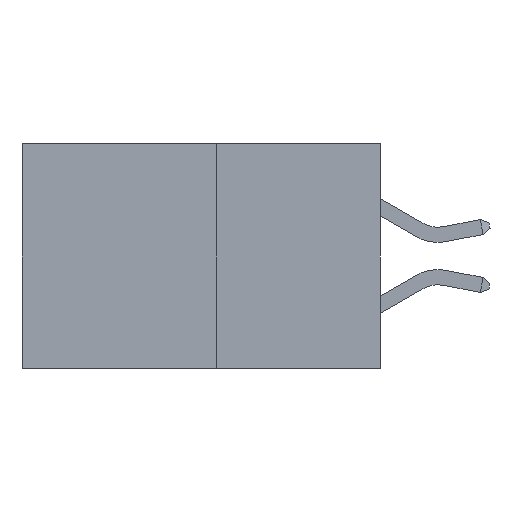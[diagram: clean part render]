
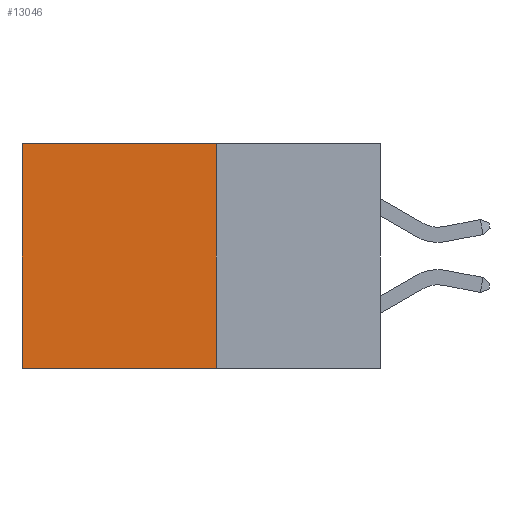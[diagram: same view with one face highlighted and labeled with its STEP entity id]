
A CAD part, left-side view. The second image highlights one B-rep face of the part: STEP entity #13046.
In plain terms, the highlighted planar face has unit normal (-1, 0, 0).
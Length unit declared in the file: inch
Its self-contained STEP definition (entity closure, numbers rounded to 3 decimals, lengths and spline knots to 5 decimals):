
#622 = LINE ( 'NONE', #9996, #13146 ) ;
#1147 = DIRECTION ( 'NONE',  ( 0., 0., -1. ) ) ;
#2276 = AXIS2_PLACEMENT_3D ( 'NONE', #18477, #28345, #23490 ) ;
#3434 = CARTESIAN_POINT ( 'NONE',  ( 0.277, 0.59, -0.37 ) ) ;
#4734 = VECTOR ( 'NONE', #1147, 39.37008 ) ;
#7025 = VERTEX_POINT ( 'NONE', #16132 ) ;
#7640 = ORIENTED_EDGE ( 'NONE', *, *, #30612, .F. ) ;
#9273 = CARTESIAN_POINT ( 'NONE',  ( 0.277, 0.27, 0. ) ) ;
#9689 = VERTEX_POINT ( 'NONE', #9793 ) ;
#9793 = CARTESIAN_POINT ( 'NONE',  ( 0.277, 0.59, 0. ) ) ;
#9996 = CARTESIAN_POINT ( 'NONE',  ( 0.277, 0.27, -0.37 ) ) ;
#10485 = CARTESIAN_POINT ( 'NONE',  ( 0.277, 0.27, 0. ) ) ;
#10578 = LINE ( 'NONE', #31014, #4734 ) ;
#10938 = VERTEX_POINT ( 'NONE', #10485 ) ;
#11768 = DIRECTION ( 'NONE',  ( 0., 1., 0. ) ) ;
#12288 = FACE_OUTER_BOUND ( 'NONE', #29305, .T. ) ;
#13046 = ADVANCED_FACE ( 'NONE', ( #12288 ), #20979, .F. ) ;
#13146 = VECTOR ( 'NONE', #29917, 39.37008 ) ;
#13270 = EDGE_CURVE ( 'NONE', #10938, #9689, #20118, .T. ) ;
#13619 = VECTOR ( 'NONE', #18523, 39.37008 ) ;
#14607 = VERTEX_POINT ( 'NONE', #27495 ) ;
#16132 = CARTESIAN_POINT ( 'NONE',  ( 0.277, 0.59, -0.37 ) ) ;
#18477 = CARTESIAN_POINT ( 'NONE',  ( 0.277, 0.27, -0.37 ) ) ;
#18523 = DIRECTION ( 'NONE',  ( 0., 0., -1. ) ) ;
#20118 = LINE ( 'NONE', #9273, #31751 ) ;
#20289 = LINE ( 'NONE', #3434, #13619 ) ;
#20979 = PLANE ( 'NONE',  #2276 ) ;
#23490 = DIRECTION ( 'NONE',  ( 0., 0., -1. ) ) ;
#26141 = ORIENTED_EDGE ( 'NONE', *, *, #13270, .T. ) ;
#27219 = EDGE_CURVE ( 'NONE', #9689, #7025, #20289, .T. ) ;
#27495 = CARTESIAN_POINT ( 'NONE',  ( 0.277, 0.27, -0.37 ) ) ;
#28018 = ORIENTED_EDGE ( 'NONE', *, *, #27219, .T. ) ;
#28345 = DIRECTION ( 'NONE',  ( 1., 0., 0. ) ) ;
#28771 = ORIENTED_EDGE ( 'NONE', *, *, #29011, .F. ) ;
#29011 = EDGE_CURVE ( 'NONE', #14607, #7025, #622, .T. ) ;
#29305 = EDGE_LOOP ( 'NONE', ( #28018, #28771, #7640, #26141 ) ) ;
#29917 = DIRECTION ( 'NONE',  ( 0., 1., 0. ) ) ;
#30612 = EDGE_CURVE ( 'NONE', #10938, #14607, #10578, .T. ) ;
#31014 = CARTESIAN_POINT ( 'NONE',  ( 0.277, 0.27, -0.37 ) ) ;
#31751 = VECTOR ( 'NONE', #11768, 39.37008 ) ;
